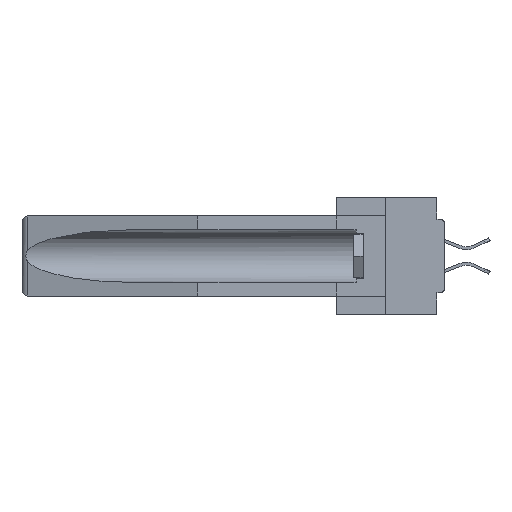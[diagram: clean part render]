
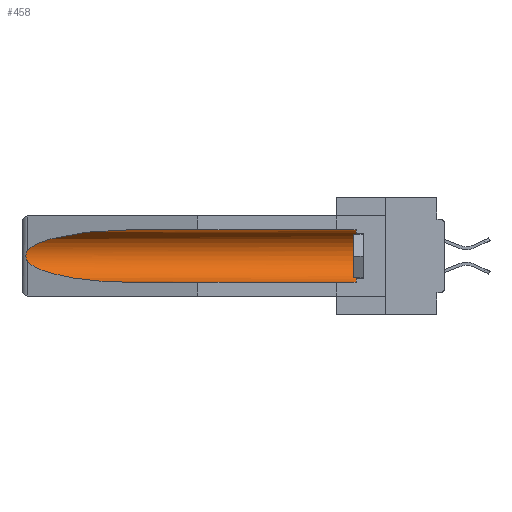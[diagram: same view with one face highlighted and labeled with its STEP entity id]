
A CAD part, left-side view. The second image highlights one B-rep face of the part: STEP entity #458.
In plain terms, the highlighted cylindrical face has radius 2.857 mm (diameter 5.715 mm), a partial arc.
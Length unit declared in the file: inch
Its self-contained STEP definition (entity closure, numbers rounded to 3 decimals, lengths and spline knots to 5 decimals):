
#458 = ADVANCED_FACE ( 'NONE', ( #17565 ), #16714, .F. ) ;
#1172 = CARTESIAN_POINT ( 'NONE',  ( 0.2673, 1.5327, -0.16383 ) ) ;
#1273 = CARTESIAN_POINT ( 'NONE',  ( 0.2675, 1.53308, -0.16763 ) ) ;
#1387 = VECTOR ( 'NONE', #30823, 39.37008 ) ;
#2999 = LINE ( 'NONE', #28628, #35217 ) ;
#3474 = CARTESIAN_POINT ( 'NONE',  ( 0.155, 1.07973, -0.059 ) ) ;
#3791 = DIRECTION ( 'NONE',  ( 0., 1., 0. ) ) ;
#4008 = VERTEX_POINT ( 'NONE', #15111 ) ;
#4022 = LINE ( 'NONE', #22304, #1387 ) ;
#4072 = CARTESIAN_POINT ( 'NONE',  ( 0.155, 0.126, -0.059 ) ) ;
#4084 = CARTESIAN_POINT ( 'NONE',  ( 0.2673, 1.53269, -0.17917 ) ) ;
#4401 = EDGE_CURVE ( 'NONE', #4008, #23028, #19501, .T. ) ;
#5041 = CARTESIAN_POINT ( 'NONE',  ( 0.155, 0.126, -0.284 ) ) ;
#5697 = EDGE_CURVE ( 'NONE', #25693, #8288, #14205, .T. ) ;
#5987 = CARTESIAN_POINT ( 'NONE',  ( 0.25451, 1.48313, -0.09465 ) ) ;
#6539 = DIRECTION ( 'NONE',  ( 0., 1., 0. ) ) ;
#6974 = CARTESIAN_POINT ( 'NONE',  ( 0.155, 1.07973, -0.284 ) ) ;
#8288 = VERTEX_POINT ( 'NONE', #4072 ) ;
#8738 = CARTESIAN_POINT ( 'NONE',  ( 0.26537, 1.52718, -0.14972 ) ) ;
#9050 = CARTESIAN_POINT ( 'NONE',  ( 0.155, -0.30754, -0.1715 ) ) ;
#9386 = EDGE_CURVE ( 'NONE', #8288, #4008, #4022, .T. ) ;
#10040 = VERTEX_POINT ( 'NONE', #33921 ) ;
#11704 = EDGE_CURVE ( 'NONE', #25693, #26540, #2999, .T. ) ;
#11798 = AXIS2_PLACEMENT_3D ( 'NONE', #23334, #14827, #12495 ) ;
#12495 = DIRECTION ( 'NONE',  ( 0., 0., 1. ) ) ;
#14205 = CIRCLE ( 'NONE', #11798, 0.1125 ) ;
#14827 = DIRECTION ( 'NONE',  ( 0., -1., 0. ) ) ;
#15091 = CARTESIAN_POINT ( 'NONE',  ( 0.25451, 1.48313, -0.24835 ) ) ;
#15111 = CARTESIAN_POINT ( 'NONE',  ( 0.155, 1.07973, -0.059 ) ) ;
#15115 = CARTESIAN_POINT ( 'NONE',  ( 0.26597, 1.5296, -0.19026 ) ) ;
#15290 =( BOUNDED_CURVE ( )  B_SPLINE_CURVE ( 3, ( #28342, #15091, #26136, #34338 ),
 .UNSPECIFIED., .F., .F. ) 
 B_SPLINE_CURVE_WITH_KNOTS ( ( 4, 4 ),
 ( 0.1948, 1.5708 ),
 .UNSPECIFIED. ) 
 CURVE ( )  GEOMETRIC_REPRESENTATION_ITEM ( )  RATIONAL_B_SPLINE_CURVE ( ( 1., 0.848, 0.848, 1. ) ) 
 REPRESENTATION_ITEM ( '' )  );
#16349 = ORIENTED_EDGE ( 'NONE', *, *, #4401, .T. ) ;
#16714 = CYLINDRICAL_SURFACE ( 'NONE', #34807, 0.1125 ) ;
#17565 = FACE_OUTER_BOUND ( 'NONE', #25425, .T. ) ;
#17948 = B_SPLINE_CURVE_WITH_KNOTS ( 'NONE', 3,
 ( #31581, #31244, #23522, #1172, #1273, #23078, #4084, #20434, #15115, #20779 ),
 .UNSPECIFIED., .F., .F.,
 ( 4, 2, 2, 2, 4 ),
 ( 0., 0.00029, 0.00058, 0.00087, 0.00117 ),
 .UNSPECIFIED. ) ;
#19289 = ORIENTED_EDGE ( 'NONE', *, *, #33914, .T. ) ;
#19501 =( BOUNDED_CURVE ( )  B_SPLINE_CURVE ( 3, ( #3474, #25195, #5987, #8738 ),
 .UNSPECIFIED., .F., .F. ) 
 B_SPLINE_CURVE_WITH_KNOTS ( ( 4, 4 ),
 ( 4.71239, 6.08839 ),
 .UNSPECIFIED. ) 
 CURVE ( )  GEOMETRIC_REPRESENTATION_ITEM ( )  RATIONAL_B_SPLINE_CURVE ( ( 1., 0.848, 0.848, 1. ) ) 
 REPRESENTATION_ITEM ( '' )  );
#20434 = CARTESIAN_POINT ( 'NONE',  ( 0.26655, 1.53094, -0.18657 ) ) ;
#20779 = CARTESIAN_POINT ( 'NONE',  ( 0.26537, 1.52718, -0.19328 ) ) ;
#22304 = CARTESIAN_POINT ( 'NONE',  ( 0.155, -0.30754, -0.059 ) ) ;
#22994 = DIRECTION ( 'NONE',  ( 0., 0., 1. ) ) ;
#23028 = VERTEX_POINT ( 'NONE', #30376 ) ;
#23078 = CARTESIAN_POINT ( 'NONE',  ( 0.2675, 1.53308, -0.17534 ) ) ;
#23334 = CARTESIAN_POINT ( 'NONE',  ( 0.155, 0.126, -0.1715 ) ) ;
#23522 = CARTESIAN_POINT ( 'NONE',  ( 0.26654, 1.53092, -0.15636 ) ) ;
#25195 = CARTESIAN_POINT ( 'NONE',  ( 0.21114, 1.30732, -0.059 ) ) ;
#25425 = EDGE_LOOP ( 'NONE', ( #16349, #30227, #19289, #26181, #27754, #31563 ) ) ;
#25693 = VERTEX_POINT ( 'NONE', #5041 ) ;
#26136 = CARTESIAN_POINT ( 'NONE',  ( 0.21114, 1.30732, -0.284 ) ) ;
#26181 = ORIENTED_EDGE ( 'NONE', *, *, #11704, .F. ) ;
#26540 = VERTEX_POINT ( 'NONE', #6974 ) ;
#27754 = ORIENTED_EDGE ( 'NONE', *, *, #5697, .T. ) ;
#28342 = CARTESIAN_POINT ( 'NONE',  ( 0.26537, 1.52718, -0.19328 ) ) ;
#28628 = CARTESIAN_POINT ( 'NONE',  ( 0.155, -0.30754, -0.284 ) ) ;
#30227 = ORIENTED_EDGE ( 'NONE', *, *, #32082, .T. ) ;
#30376 = CARTESIAN_POINT ( 'NONE',  ( 0.26537, 1.52718, -0.14972 ) ) ;
#30823 = DIRECTION ( 'NONE',  ( 0., 1., 0. ) ) ;
#31244 = CARTESIAN_POINT ( 'NONE',  ( 0.26597, 1.52961, -0.15275 ) ) ;
#31563 = ORIENTED_EDGE ( 'NONE', *, *, #9386, .T. ) ;
#31581 = CARTESIAN_POINT ( 'NONE',  ( 0.26537, 1.52718, -0.14972 ) ) ;
#32082 = EDGE_CURVE ( 'NONE', #23028, #10040, #17948, .T. ) ;
#33914 = EDGE_CURVE ( 'NONE', #10040, #26540, #15290, .T. ) ;
#33921 = CARTESIAN_POINT ( 'NONE',  ( 0.26537, 1.52718, -0.19328 ) ) ;
#34338 = CARTESIAN_POINT ( 'NONE',  ( 0.155, 1.07973, -0.284 ) ) ;
#34807 = AXIS2_PLACEMENT_3D ( 'NONE', #9050, #3791, #22994 ) ;
#35217 = VECTOR ( 'NONE', #6539, 39.37008 ) ;
